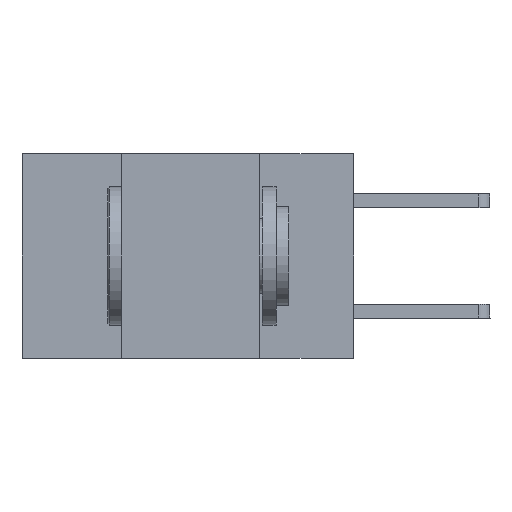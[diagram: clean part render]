
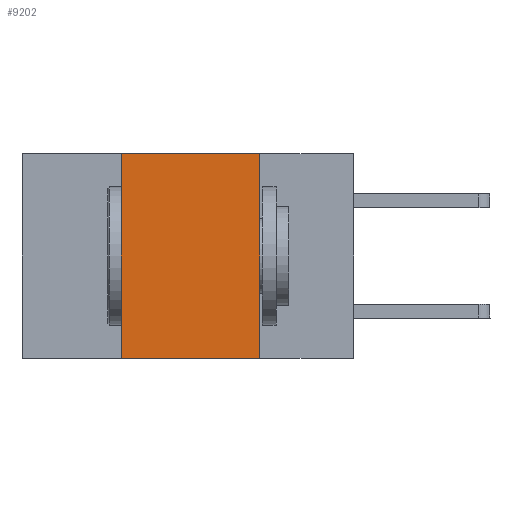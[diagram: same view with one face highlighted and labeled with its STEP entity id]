
A CAD part, left-side view. The second image highlights one B-rep face of the part: STEP entity #9202.
In plain terms, the highlighted planar face has unit normal (-1, 0, 0).
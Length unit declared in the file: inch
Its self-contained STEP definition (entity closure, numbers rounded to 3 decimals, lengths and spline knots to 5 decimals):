
#783 = PLANE ( 'NONE',  #3276 ) ;
#823 = VERTEX_POINT ( 'NONE', #1455 ) ;
#905 = EDGE_LOOP ( 'NONE', ( #7415, #5798, #2333, #3688 ) ) ;
#933 = VERTEX_POINT ( 'NONE', #5718 ) ;
#1455 = CARTESIAN_POINT ( 'NONE',  ( 0., 0.17, 0. ) ) ;
#2181 = CARTESIAN_POINT ( 'NONE',  ( 0., 0.6, -0.37 ) ) ;
#2333 = ORIENTED_EDGE ( 'NONE', *, *, #10285, .F. ) ;
#2543 = LINE ( 'NONE', #2181, #5383 ) ;
#2775 = CARTESIAN_POINT ( 'NONE',  ( 0., 0.42, 0. ) ) ;
#2806 = CARTESIAN_POINT ( 'NONE',  ( 0., 0.6, 0. ) ) ;
#3276 = AXIS2_PLACEMENT_3D ( 'NONE', #2806, #5641, #12063 ) ;
#3392 = FACE_OUTER_BOUND ( 'NONE', #905, .T. ) ;
#3688 = ORIENTED_EDGE ( 'NONE', *, *, #6353, .T. ) ;
#3842 = CARTESIAN_POINT ( 'NONE',  ( 0., 0.17, 0. ) ) ;
#4400 = VECTOR ( 'NONE', #8380, 39.37008 ) ;
#4723 = CARTESIAN_POINT ( 'NONE',  ( 0., 0.17, -0.37 ) ) ;
#4798 = DIRECTION ( 'NONE',  ( 0., 0., -1. ) ) ;
#5383 = VECTOR ( 'NONE', #8710, 39.37008 ) ;
#5641 = DIRECTION ( 'NONE',  ( 1., 0., 0. ) ) ;
#5718 = CARTESIAN_POINT ( 'NONE',  ( 0., 0.42, -0.37 ) ) ;
#5798 = ORIENTED_EDGE ( 'NONE', *, *, #11450, .F. ) ;
#6166 = VERTEX_POINT ( 'NONE', #4723 ) ;
#6353 = EDGE_CURVE ( 'NONE', #933, #6166, #2543, .T. ) ;
#7415 = ORIENTED_EDGE ( 'NONE', *, *, #11489, .F. ) ;
#7440 = CARTESIAN_POINT ( 'NONE',  ( 0., 0.6, 0. ) ) ;
#8150 = VECTOR ( 'NONE', #9320, 39.37008 ) ;
#8380 = DIRECTION ( 'NONE',  ( 0., -1., 0. ) ) ;
#8639 = CARTESIAN_POINT ( 'NONE',  ( 0., 0.42, 0. ) ) ;
#8650 = VERTEX_POINT ( 'NONE', #8639 ) ;
#8702 = VECTOR ( 'NONE', #4798, 39.37008 ) ;
#8710 = DIRECTION ( 'NONE',  ( 0., -1., 0. ) ) ;
#8987 = LINE ( 'NONE', #3842, #8702 ) ;
#9202 = ADVANCED_FACE ( 'NONE', ( #3392 ), #783, .F. ) ;
#9320 = DIRECTION ( 'NONE',  ( 0., 0., 1. ) ) ;
#10285 = EDGE_CURVE ( 'NONE', #933, #8650, #10692, .T. ) ;
#10692 = LINE ( 'NONE', #2775, #8150 ) ;
#11450 = EDGE_CURVE ( 'NONE', #8650, #823, #11728, .T. ) ;
#11489 = EDGE_CURVE ( 'NONE', #823, #6166, #8987, .T. ) ;
#11728 = LINE ( 'NONE', #7440, #4400 ) ;
#12063 = DIRECTION ( 'NONE',  ( 0., 0., -1. ) ) ;
